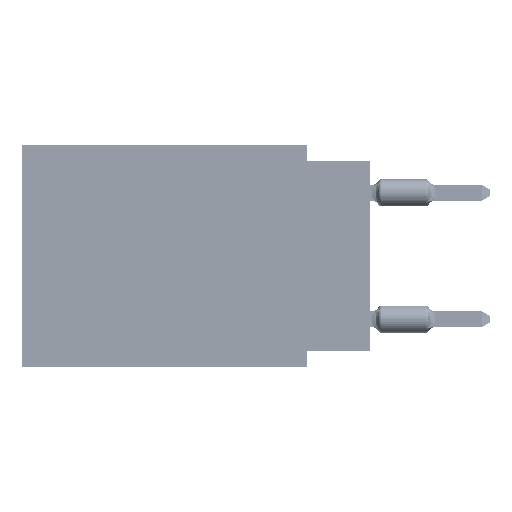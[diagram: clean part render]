
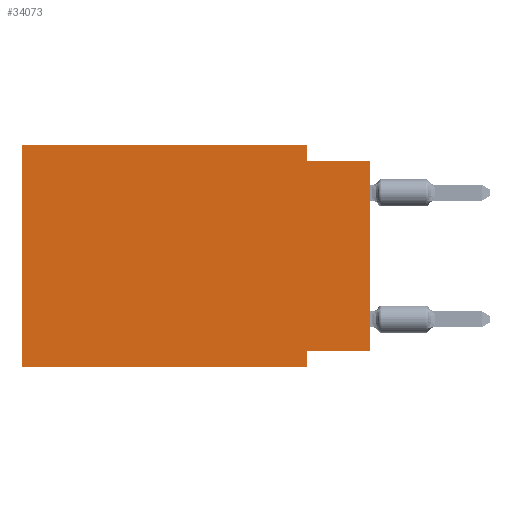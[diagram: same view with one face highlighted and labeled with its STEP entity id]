
A CAD part, left-side view. The second image highlights one B-rep face of the part: STEP entity #34073.
In plain terms, the highlighted planar face has unit normal (-1, 0, 0).
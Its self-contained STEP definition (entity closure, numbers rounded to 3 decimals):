
#18 = LINE ( 'NONE', #32067, #26857 ) ;
#1464 = LINE ( 'NONE', #71488, #69876 ) ;
#2167 = CARTESIAN_POINT ( 'NONE',  ( 0., 13.97, -8.89 ) ) ;
#2951 = CARTESIAN_POINT ( 'NONE',  ( 0., 0., -0.635 ) ) ;
#3889 = CARTESIAN_POINT ( 'NONE',  ( 0., 0., 0. ) ) ;
#4816 = EDGE_CURVE ( 'NONE', #28943, #50039, #60020, .T. ) ;
#7466 = VERTEX_POINT ( 'NONE', #35290 ) ;
#8968 = AXIS2_PLACEMENT_3D ( 'NONE', #13124, #12294, #76844 ) ;
#9838 = ORIENTED_EDGE ( 'NONE', *, *, #14041, .F. ) ;
#10936 = VECTOR ( 'NONE', #13408, 1000. ) ;
#12294 = DIRECTION ( 'NONE',  ( 1., 0., 0. ) ) ;
#12489 = VECTOR ( 'NONE', #77025, 1000. ) ;
#12901 = LINE ( 'NONE', #56796, #12489 ) ;
#13124 = CARTESIAN_POINT ( 'NONE',  ( 0., 13.97, 0. ) ) ;
#13408 = DIRECTION ( 'NONE',  ( 0., -1., 0. ) ) ;
#14041 = EDGE_CURVE ( 'NONE', #57051, #7466, #58704, .T. ) ;
#14276 = VERTEX_POINT ( 'NONE', #47289 ) ;
#18322 = ORIENTED_EDGE ( 'NONE', *, *, #77749, .T. ) ;
#20567 = LINE ( 'NONE', #20985, #10936 ) ;
#20985 = CARTESIAN_POINT ( 'NONE',  ( 0., 0., -0.635 ) ) ;
#21549 = LINE ( 'NONE', #2167, #62056 ) ;
#23971 = EDGE_CURVE ( 'NONE', #59043, #24761, #18, .T. ) ;
#24761 = VERTEX_POINT ( 'NONE', #42884 ) ;
#25189 = VERTEX_POINT ( 'NONE', #51901 ) ;
#25424 = CARTESIAN_POINT ( 'NONE',  ( 0., 2.54, 0. ) ) ;
#26648 = DIRECTION ( 'NONE',  ( 0., 0., -1. ) ) ;
#26857 = VECTOR ( 'NONE', #39240, 1000. ) ;
#26991 = ORIENTED_EDGE ( 'NONE', *, *, #29413, .F. ) ;
#27914 = EDGE_CURVE ( 'NONE', #24761, #50039, #20567, .T. ) ;
#28943 = VERTEX_POINT ( 'NONE', #73070 ) ;
#29413 = EDGE_CURVE ( 'NONE', #28943, #57051, #12901, .T. ) ;
#32067 = CARTESIAN_POINT ( 'NONE',  ( 0., 2.54, 0. ) ) ;
#33922 = DIRECTION ( 'NONE',  ( 0., -1., 0. ) ) ;
#34073 = ADVANCED_FACE ( 'NONE', ( #51096 ), #82329, .F. ) ;
#35290 = CARTESIAN_POINT ( 'NONE',  ( 0., 2.54, -8.89 ) ) ;
#39240 = DIRECTION ( 'NONE',  ( 0., 0., -1. ) ) ;
#39699 = EDGE_LOOP ( 'NONE', ( #61613, #74573, #58329, #40648, #52741, #18322, #9838, #26991 ) ) ;
#40648 = ORIENTED_EDGE ( 'NONE', *, *, #41343, .F. ) ;
#41343 = EDGE_CURVE ( 'NONE', #25189, #59043, #1464, .T. ) ;
#41925 = VECTOR ( 'NONE', #64099, 1000. ) ;
#42884 = CARTESIAN_POINT ( 'NONE',  ( 0., 2.54, -0.635 ) ) ;
#44687 = LINE ( 'NONE', #64939, #41925 ) ;
#47289 = CARTESIAN_POINT ( 'NONE',  ( 0., 13.97, -8.89 ) ) ;
#47852 = VECTOR ( 'NONE', #48620, 1000. ) ;
#48620 = DIRECTION ( 'NONE',  ( 0., 0., 1. ) ) ;
#50039 = VERTEX_POINT ( 'NONE', #2951 ) ;
#51096 = FACE_OUTER_BOUND ( 'NONE', #39699, .T. ) ;
#51901 = CARTESIAN_POINT ( 'NONE',  ( 0., 13.97, 0. ) ) ;
#52741 = ORIENTED_EDGE ( 'NONE', *, *, #53360, .F. ) ;
#53360 = EDGE_CURVE ( 'NONE', #14276, #25189, #44687, .T. ) ;
#56796 = CARTESIAN_POINT ( 'NONE',  ( 0., 0., -8.255 ) ) ;
#57051 = VERTEX_POINT ( 'NONE', #70994 ) ;
#58329 = ORIENTED_EDGE ( 'NONE', *, *, #23971, .F. ) ;
#58704 = LINE ( 'NONE', #65045, #76183 ) ;
#59043 = VERTEX_POINT ( 'NONE', #25424 ) ;
#60020 = LINE ( 'NONE', #3889, #47852 ) ;
#61613 = ORIENTED_EDGE ( 'NONE', *, *, #4816, .T. ) ;
#62056 = VECTOR ( 'NONE', #73444, 1000. ) ;
#64099 = DIRECTION ( 'NONE',  ( 0., 0., 1. ) ) ;
#64939 = CARTESIAN_POINT ( 'NONE',  ( 0., 13.97, 0. ) ) ;
#65045 = CARTESIAN_POINT ( 'NONE',  ( 0., 2.54, -8.89 ) ) ;
#69876 = VECTOR ( 'NONE', #33922, 1000. ) ;
#70994 = CARTESIAN_POINT ( 'NONE',  ( 0., 2.54, -8.255 ) ) ;
#71488 = CARTESIAN_POINT ( 'NONE',  ( 0., 13.97, 0. ) ) ;
#73070 = CARTESIAN_POINT ( 'NONE',  ( 0., 0., -8.255 ) ) ;
#73444 = DIRECTION ( 'NONE',  ( 0., -1., 0. ) ) ;
#74573 = ORIENTED_EDGE ( 'NONE', *, *, #27914, .F. ) ;
#76183 = VECTOR ( 'NONE', #26648, 1000. ) ;
#76844 = DIRECTION ( 'NONE',  ( 0., 0., -1. ) ) ;
#77025 = DIRECTION ( 'NONE',  ( 0., 1., 0. ) ) ;
#77749 = EDGE_CURVE ( 'NONE', #14276, #7466, #21549, .T. ) ;
#82329 = PLANE ( 'NONE',  #8968 ) ;
